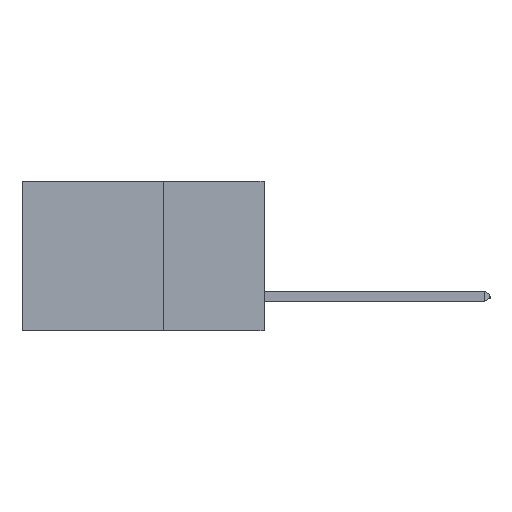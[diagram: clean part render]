
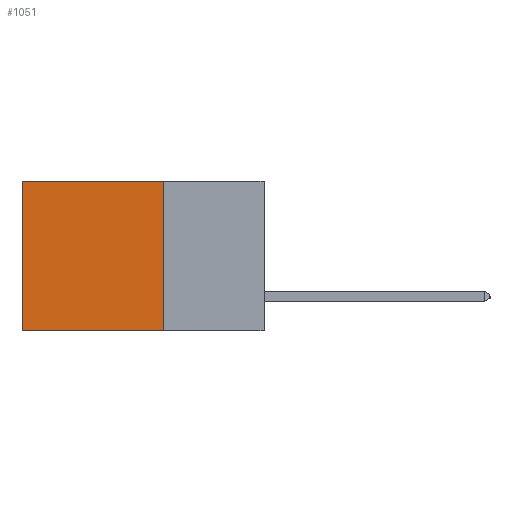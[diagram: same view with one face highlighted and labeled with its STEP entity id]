
A CAD part, left-side view. The second image highlights one B-rep face of the part: STEP entity #1051.
In plain terms, the highlighted planar face has unit normal (-1, 0, 0).
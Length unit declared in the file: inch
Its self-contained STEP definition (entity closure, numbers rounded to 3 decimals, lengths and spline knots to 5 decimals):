
#476 = LINE ( 'NONE', #9302, #13299 ) ;
#1051 = ADVANCED_FACE ( 'NONE', ( #8030 ), #19546, .F. ) ;
#1639 = VECTOR ( 'NONE', #9272, 39.37008 ) ;
#2174 = CARTESIAN_POINT ( 'NONE',  ( 0.298, 0.25, -0.37 ) ) ;
#2314 = EDGE_LOOP ( 'NONE', ( #11873, #18990, #17235, #3894 ) ) ;
#2384 = LINE ( 'NONE', #14505, #10774 ) ;
#3347 = CARTESIAN_POINT ( 'NONE',  ( 0.298, 0.6, 0. ) ) ;
#3705 = DIRECTION ( 'NONE',  ( 0., 0., -1. ) ) ;
#3894 = ORIENTED_EDGE ( 'NONE', *, *, #21011, .T. ) ;
#4224 = CARTESIAN_POINT ( 'NONE',  ( 0.298, 0.6, -0.37 ) ) ;
#6589 = EDGE_CURVE ( 'NONE', #10117, #10942, #10589, .T. ) ;
#7877 = CARTESIAN_POINT ( 'NONE',  ( 0.298, 0.25, 0. ) ) ;
#7907 = EDGE_CURVE ( 'NONE', #16457, #10942, #2384, .T. ) ;
#8030 = FACE_OUTER_BOUND ( 'NONE', #2314, .T. ) ;
#8523 = DIRECTION ( 'NONE',  ( 1., 0., 0. ) ) ;
#9272 = DIRECTION ( 'NONE',  ( 0., 1., 0. ) ) ;
#9302 = CARTESIAN_POINT ( 'NONE',  ( 0.298, 0.25, 0. ) ) ;
#10117 = VERTEX_POINT ( 'NONE', #2174 ) ;
#10220 = CARTESIAN_POINT ( 'NONE',  ( 0.298, 0.25, 0. ) ) ;
#10589 = LINE ( 'NONE', #20654, #1639 ) ;
#10774 = VECTOR ( 'NONE', #16115, 39.37008 ) ;
#10942 = VERTEX_POINT ( 'NONE', #4224 ) ;
#10973 = DIRECTION ( 'NONE',  ( 0., 1., 0. ) ) ;
#11667 = VERTEX_POINT ( 'NONE', #7877 ) ;
#11873 = ORIENTED_EDGE ( 'NONE', *, *, #7907, .T. ) ;
#11900 = DIRECTION ( 'NONE',  ( 0., 0., -1. ) ) ;
#12592 = EDGE_CURVE ( 'NONE', #11667, #10117, #16337, .T. ) ;
#12648 = CARTESIAN_POINT ( 'NONE',  ( 0.298, 0.25, 0. ) ) ;
#13299 = VECTOR ( 'NONE', #10973, 39.37008 ) ;
#14505 = CARTESIAN_POINT ( 'NONE',  ( 0.298, 0.6, 0. ) ) ;
#16115 = DIRECTION ( 'NONE',  ( 0., 0., -1. ) ) ;
#16337 = LINE ( 'NONE', #10220, #19653 ) ;
#16457 = VERTEX_POINT ( 'NONE', #3347 ) ;
#17235 = ORIENTED_EDGE ( 'NONE', *, *, #12592, .F. ) ;
#18990 = ORIENTED_EDGE ( 'NONE', *, *, #6589, .F. ) ;
#19546 = PLANE ( 'NONE',  #20385 ) ;
#19653 = VECTOR ( 'NONE', #11900, 39.37008 ) ;
#20385 = AXIS2_PLACEMENT_3D ( 'NONE', #12648, #8523, #3705 ) ;
#20654 = CARTESIAN_POINT ( 'NONE',  ( 0.298, 0.25, -0.37 ) ) ;
#21011 = EDGE_CURVE ( 'NONE', #11667, #16457, #476, .T. ) ;
